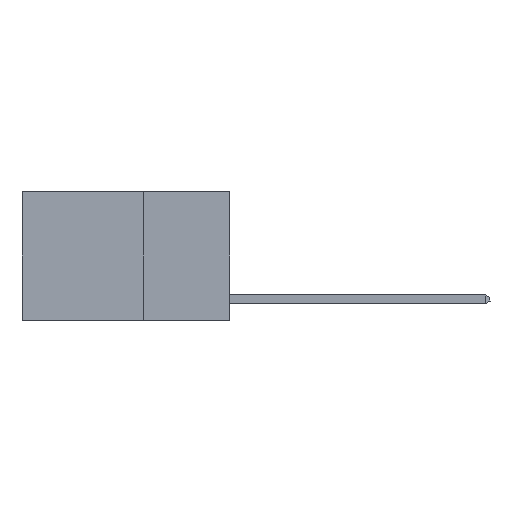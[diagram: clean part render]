
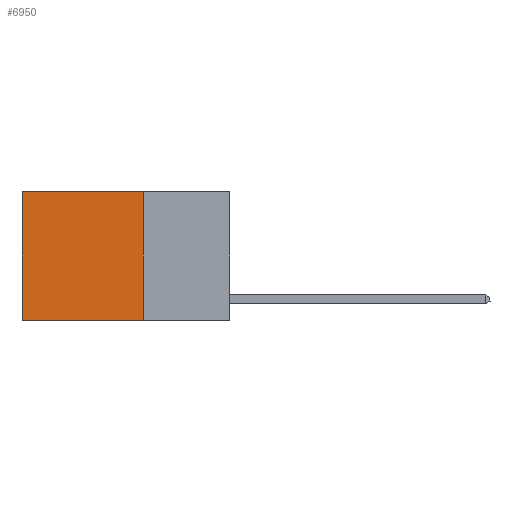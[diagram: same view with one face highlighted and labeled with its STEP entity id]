
A CAD part, left-side view. The second image highlights one B-rep face of the part: STEP entity #6950.
In plain terms, the highlighted planar face has unit normal (-1, 0, 0).
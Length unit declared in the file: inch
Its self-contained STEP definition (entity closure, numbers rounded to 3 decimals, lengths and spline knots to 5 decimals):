
#38 = DIRECTION ( 'NONE',  ( 0., 0., -1. ) ) ;
#379 = VECTOR ( 'NONE', #38, 39.37008 ) ;
#443 = DIRECTION ( 'NONE',  ( 1., 0., 0. ) ) ;
#651 = DIRECTION ( 'NONE',  ( 0., 0., -1. ) ) ;
#693 = CARTESIAN_POINT ( 'NONE',  ( 0.2625, 0.25, 0. ) ) ;
#1212 = EDGE_LOOP ( 'NONE', ( #4004, #6171, #2136, #2803 ) ) ;
#2136 = ORIENTED_EDGE ( 'NONE', *, *, #4786, .F. ) ;
#2142 = LINE ( 'NONE', #9020, #7154 ) ;
#2189 = EDGE_CURVE ( 'NONE', #9421, #10610, #7079, .T. ) ;
#2385 = FACE_OUTER_BOUND ( 'NONE', #1212, .T. ) ;
#2561 = CARTESIAN_POINT ( 'NONE',  ( 0.2625, 0.25, -0.37 ) ) ;
#2672 = CARTESIAN_POINT ( 'NONE',  ( 0.2625, 0.25, 0. ) ) ;
#2803 = ORIENTED_EDGE ( 'NONE', *, *, #10156, .T. ) ;
#2985 = AXIS2_PLACEMENT_3D ( 'NONE', #3058, #443, #9283 ) ;
#3058 = CARTESIAN_POINT ( 'NONE',  ( 0.2625, 0.25, 0. ) ) ;
#3115 = CARTESIAN_POINT ( 'NONE',  ( 0.2625, 0.6, 0. ) ) ;
#4004 = ORIENTED_EDGE ( 'NONE', *, *, #8621, .T. ) ;
#4446 = VERTEX_POINT ( 'NONE', #2672 ) ;
#4717 = PLANE ( 'NONE',  #2985 ) ;
#4786 = EDGE_CURVE ( 'NONE', #4446, #9421, #8269, .T. ) ;
#5073 = VERTEX_POINT ( 'NONE', #3115 ) ;
#6171 = ORIENTED_EDGE ( 'NONE', *, *, #2189, .F. ) ;
#6950 = ADVANCED_FACE ( 'NONE', ( #2385 ), #4717, .F. ) ;
#7079 = LINE ( 'NONE', #2561, #10973 ) ;
#7154 = VECTOR ( 'NONE', #7296, 39.37008 ) ;
#7296 = DIRECTION ( 'NONE',  ( 0., 1., 0. ) ) ;
#7938 = CARTESIAN_POINT ( 'NONE',  ( 0.2625, 0.25, -0.37 ) ) ;
#8269 = LINE ( 'NONE', #693, #10793 ) ;
#8621 = EDGE_CURVE ( 'NONE', #5073, #10610, #9394, .T. ) ;
#8792 = DIRECTION ( 'NONE',  ( 0., 1., 0. ) ) ;
#9020 = CARTESIAN_POINT ( 'NONE',  ( 0.2625, 0.25, 0. ) ) ;
#9283 = DIRECTION ( 'NONE',  ( 0., 0., -1. ) ) ;
#9394 = LINE ( 'NONE', #10630, #379 ) ;
#9421 = VERTEX_POINT ( 'NONE', #7938 ) ;
#10120 = CARTESIAN_POINT ( 'NONE',  ( 0.2625, 0.6, -0.37 ) ) ;
#10156 = EDGE_CURVE ( 'NONE', #4446, #5073, #2142, .T. ) ;
#10610 = VERTEX_POINT ( 'NONE', #10120 ) ;
#10630 = CARTESIAN_POINT ( 'NONE',  ( 0.2625, 0.6, 0. ) ) ;
#10793 = VECTOR ( 'NONE', #651, 39.37008 ) ;
#10973 = VECTOR ( 'NONE', #8792, 39.37008 ) ;
